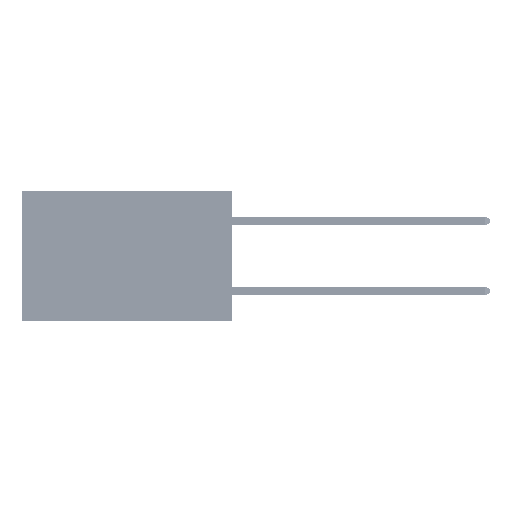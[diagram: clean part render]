
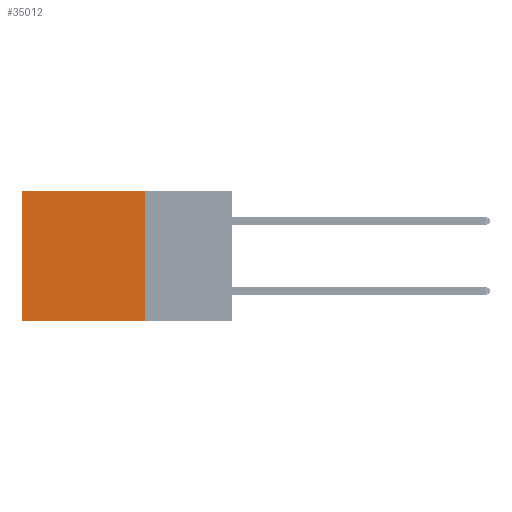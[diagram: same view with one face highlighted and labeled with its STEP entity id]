
A CAD part, left-side view. The second image highlights one B-rep face of the part: STEP entity #35012.
In plain terms, the highlighted planar face has unit normal (-1, 0, 0).
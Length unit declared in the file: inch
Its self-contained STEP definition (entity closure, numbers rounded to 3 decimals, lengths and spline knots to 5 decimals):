
#459 = CARTESIAN_POINT ( 'NONE',  ( 0.2875, 0.6, 0. ) ) ;
#2007 = CARTESIAN_POINT ( 'NONE',  ( 0.2875, 0.6, 0. ) ) ;
#2466 = EDGE_CURVE ( 'NONE', #13616, #23237, #40255, .T. ) ;
#2709 = VERTEX_POINT ( 'NONE', #3799 ) ;
#3156 = ORIENTED_EDGE ( 'NONE', *, *, #2466, .T. ) ;
#3799 = CARTESIAN_POINT ( 'NONE',  ( 0.2875, 0.6, -0.37 ) ) ;
#4026 = VERTEX_POINT ( 'NONE', #28567 ) ;
#4213 = LINE ( 'NONE', #33621, #10629 ) ;
#4586 = CARTESIAN_POINT ( 'NONE',  ( 0.2875, 0.25, 0. ) ) ;
#5193 = CARTESIAN_POINT ( 'NONE',  ( 0.2875, 0.25, 0. ) ) ;
#8724 = ORIENTED_EDGE ( 'NONE', *, *, #24860, .F. ) ;
#9658 = DIRECTION ( 'NONE',  ( 0., 0., -1. ) ) ;
#10048 = EDGE_CURVE ( 'NONE', #13616, #4026, #4213, .T. ) ;
#10066 = DIRECTION ( 'NONE',  ( 0., 0., -1. ) ) ;
#10629 = VECTOR ( 'NONE', #9658, 39.37008 ) ;
#13333 = DIRECTION ( 'NONE',  ( 1., 0., 0. ) ) ;
#13616 = VERTEX_POINT ( 'NONE', #4586 ) ;
#13950 = LINE ( 'NONE', #2007, #19708 ) ;
#17342 = EDGE_LOOP ( 'NONE', ( #24226, #8724, #39663, #3156 ) ) ;
#19708 = VECTOR ( 'NONE', #10066, 39.37008 ) ;
#20315 = VECTOR ( 'NONE', #47570, 39.37008 ) ;
#20945 = DIRECTION ( 'NONE',  ( 0., 1., 0. ) ) ;
#21401 = DIRECTION ( 'NONE',  ( 0., 0., -1. ) ) ;
#23237 = VERTEX_POINT ( 'NONE', #459 ) ;
#24226 = ORIENTED_EDGE ( 'NONE', *, *, #24268, .T. ) ;
#24268 = EDGE_CURVE ( 'NONE', #23237, #2709, #13950, .T. ) ;
#24860 = EDGE_CURVE ( 'NONE', #4026, #2709, #30544, .T. ) ;
#25770 = AXIS2_PLACEMENT_3D ( 'NONE', #29273, #13333, #21401 ) ;
#28567 = CARTESIAN_POINT ( 'NONE',  ( 0.2875, 0.25, -0.37 ) ) ;
#29273 = CARTESIAN_POINT ( 'NONE',  ( 0.2875, 0.25, 0. ) ) ;
#29276 = VECTOR ( 'NONE', #20945, 39.37008 ) ;
#30544 = LINE ( 'NONE', #39339, #20315 ) ;
#33621 = CARTESIAN_POINT ( 'NONE',  ( 0.2875, 0.25, 0. ) ) ;
#35012 = ADVANCED_FACE ( 'NONE', ( #39804 ), #37857, .F. ) ;
#37857 = PLANE ( 'NONE',  #25770 ) ;
#39339 = CARTESIAN_POINT ( 'NONE',  ( 0.2875, 0.25, -0.37 ) ) ;
#39663 = ORIENTED_EDGE ( 'NONE', *, *, #10048, .F. ) ;
#39804 = FACE_OUTER_BOUND ( 'NONE', #17342, .T. ) ;
#40255 = LINE ( 'NONE', #5193, #29276 ) ;
#47570 = DIRECTION ( 'NONE',  ( 0., 1., 0. ) ) ;
